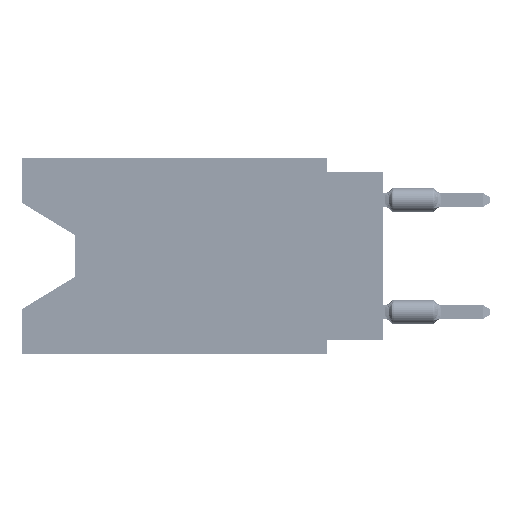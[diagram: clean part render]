
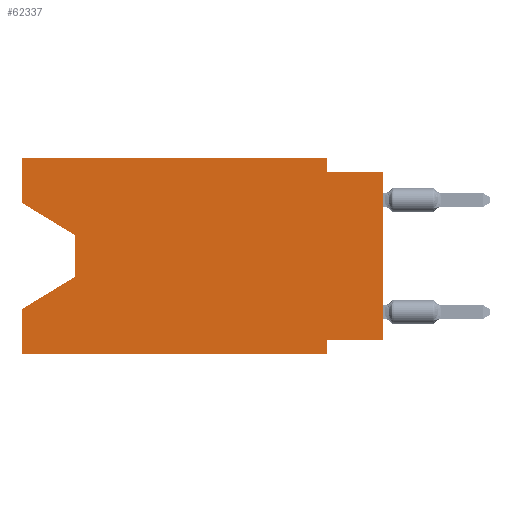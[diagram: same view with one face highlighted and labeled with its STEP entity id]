
A CAD part, left-side view. The second image highlights one B-rep face of the part: STEP entity #62337.
In plain terms, the highlighted planar face has unit normal (-1, 0, 0).
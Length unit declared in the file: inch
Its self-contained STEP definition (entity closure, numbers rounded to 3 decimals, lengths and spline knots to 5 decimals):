
#1191 = ORIENTED_EDGE ( 'NONE', *, *, #23479, .F. ) ;
#1272 = DIRECTION ( 'NONE',  ( 0., -1., 0. ) ) ;
#1857 = LINE ( 'NONE', #12989, #27364 ) ;
#2839 = LINE ( 'NONE', #30443, #30662 ) ;
#3334 = ORIENTED_EDGE ( 'NONE', *, *, #30264, .T. ) ;
#4601 = VECTOR ( 'NONE', #22509, 39.37008 ) ;
#4722 = DIRECTION ( 'NONE',  ( 0., 0., 1. ) ) ;
#5145 = ORIENTED_EDGE ( 'NONE', *, *, #39439, .F. ) ;
#5675 = CARTESIAN_POINT ( 'NONE',  ( 0., 0.55, -0.138 ) ) ;
#5821 = ORIENTED_EDGE ( 'NONE', *, *, #44535, .T. ) ;
#6218 = EDGE_CURVE ( 'NONE', #67840, #54219, #1857, .T. ) ;
#6361 = LINE ( 'NONE', #37998, #4601 ) ;
#7333 = LINE ( 'NONE', #46051, #47395 ) ;
#7729 = DIRECTION ( 'NONE',  ( 0., 0.855, -0.519 ) ) ;
#7943 = VECTOR ( 'NONE', #45613, 39.37008 ) ;
#8636 = LINE ( 'NONE', #47024, #56305 ) ;
#8919 = DIRECTION ( 'NONE',  ( 0., -1., 0. ) ) ;
#9438 = VERTEX_POINT ( 'NONE', #67692 ) ;
#9971 = ORIENTED_EDGE ( 'NONE', *, *, #41103, .F. ) ;
#10302 = CARTESIAN_POINT ( 'NONE',  ( 0., 0.1, -0.325 ) ) ;
#11143 = VECTOR ( 'NONE', #7729, 39.37008 ) ;
#12989 = CARTESIAN_POINT ( 'NONE',  ( 0., 0., -0.025 ) ) ;
#14322 = CARTESIAN_POINT ( 'NONE',  ( 0., 0.645, 0. ) ) ;
#14643 = CARTESIAN_POINT ( 'NONE',  ( 0., 0.1, -0.025 ) ) ;
#18408 = CARTESIAN_POINT ( 'NONE',  ( 0., 0.645, -0.08025 ) ) ;
#19394 = VERTEX_POINT ( 'NONE', #65000 ) ;
#20054 = DIRECTION ( 'NONE',  ( 0., 0., -1. ) ) ;
#21131 = CARTESIAN_POINT ( 'NONE',  ( 0., 0.1, 0. ) ) ;
#21195 = LINE ( 'NONE', #63802, #25116 ) ;
#21455 = LINE ( 'NONE', #53356, #33268 ) ;
#22118 = VERTEX_POINT ( 'NONE', #34055 ) ;
#22509 = DIRECTION ( 'NONE',  ( 0., 1., 0. ) ) ;
#23479 = EDGE_CURVE ( 'NONE', #62918, #26682, #6361, .T. ) ;
#23802 = CARTESIAN_POINT ( 'NONE',  ( 0., 0.645, 0. ) ) ;
#25116 = VECTOR ( 'NONE', #4722, 39.37008 ) ;
#26682 = VERTEX_POINT ( 'NONE', #10302 ) ;
#27364 = VECTOR ( 'NONE', #29454, 39.37008 ) ;
#29143 = EDGE_CURVE ( 'NONE', #19394, #67840, #36161, .T. ) ;
#29362 = VECTOR ( 'NONE', #67140, 39.37008 ) ;
#29454 = DIRECTION ( 'NONE',  ( 0., -1., 0. ) ) ;
#29942 = VERTEX_POINT ( 'NONE', #64308 ) ;
#30114 = DIRECTION ( 'NONE',  ( 0., 0., -1. ) ) ;
#30264 = EDGE_CURVE ( 'NONE', #40024, #62748, #2839, .T. ) ;
#30443 = CARTESIAN_POINT ( 'NONE',  ( 0., 0.645, -0.35 ) ) ;
#30662 = VECTOR ( 'NONE', #8919, 39.37008 ) ;
#31284 = ORIENTED_EDGE ( 'NONE', *, *, #58803, .F. ) ;
#32242 = CARTESIAN_POINT ( 'NONE',  ( 0., 0.645, -0.35 ) ) ;
#32249 = DIRECTION ( 'NONE',  ( 0., 0., -1. ) ) ;
#33268 = VECTOR ( 'NONE', #20054, 39.37008 ) ;
#33878 = VERTEX_POINT ( 'NONE', #5675 ) ;
#34055 = CARTESIAN_POINT ( 'NONE',  ( 0., 0.645, 0. ) ) ;
#34913 = LINE ( 'NONE', #23802, #58623 ) ;
#36161 = LINE ( 'NONE', #21131, #68296 ) ;
#36640 = DIRECTION ( 'NONE',  ( 0., 0., -1. ) ) ;
#37501 = ORIENTED_EDGE ( 'NONE', *, *, #63225, .F. ) ;
#37891 = ORIENTED_EDGE ( 'NONE', *, *, #43402, .T. ) ;
#37998 = CARTESIAN_POINT ( 'NONE',  ( 0., 0., -0.325 ) ) ;
#39260 = LINE ( 'NONE', #61077, #29362 ) ;
#39439 = EDGE_CURVE ( 'NONE', #40024, #61626, #21195, .T. ) ;
#40024 = VERTEX_POINT ( 'NONE', #32242 ) ;
#41103 = EDGE_CURVE ( 'NONE', #26682, #62748, #21455, .T. ) ;
#42375 = EDGE_CURVE ( 'NONE', #33878, #29942, #8636, .T. ) ;
#43402 = EDGE_CURVE ( 'NONE', #62918, #54219, #39260, .T. ) ;
#44535 = EDGE_CURVE ( 'NONE', #29942, #61626, #46114, .T. ) ;
#45613 = DIRECTION ( 'NONE',  ( 0., -0.855, -0.519 ) ) ;
#46051 = CARTESIAN_POINT ( 'NONE',  ( 0., 0.645, 0. ) ) ;
#46114 = LINE ( 'NONE', #53506, #11143 ) ;
#46610 = EDGE_LOOP ( 'NONE', ( #55899, #56020, #5821, #5145, #3334, #9971, #1191, #37891, #53678, #57524, #31284, #37501 ) ) ;
#47024 = CARTESIAN_POINT ( 'NONE',  ( 0., 0.55, -0.138 ) ) ;
#47395 = VECTOR ( 'NONE', #1272, 39.37008 ) ;
#51102 = CARTESIAN_POINT ( 'NONE',  ( 0., 0.1, -0.35 ) ) ;
#51712 = LINE ( 'NONE', #18408, #7943 ) ;
#51755 = DIRECTION ( 'NONE',  ( 0., 0., 1. ) ) ;
#53356 = CARTESIAN_POINT ( 'NONE',  ( 0., 0.1, -0.35 ) ) ;
#53506 = CARTESIAN_POINT ( 'NONE',  ( 0., 0.55, -0.212 ) ) ;
#53678 = ORIENTED_EDGE ( 'NONE', *, *, #6218, .F. ) ;
#54219 = VERTEX_POINT ( 'NONE', #67695 ) ;
#55899 = ORIENTED_EDGE ( 'NONE', *, *, #66249, .T. ) ;
#56020 = ORIENTED_EDGE ( 'NONE', *, *, #42375, .T. ) ;
#56305 = VECTOR ( 'NONE', #36640, 39.37008 ) ;
#57524 = ORIENTED_EDGE ( 'NONE', *, *, #29143, .F. ) ;
#57679 = DIRECTION ( 'NONE',  ( 1., 0., 0. ) ) ;
#58623 = VECTOR ( 'NONE', #51755, 39.37008 ) ;
#58761 = PLANE ( 'NONE',  #68171 ) ;
#58803 = EDGE_CURVE ( 'NONE', #22118, #19394, #7333, .T. ) ;
#59719 = CARTESIAN_POINT ( 'NONE',  ( 0., 0., -0.325 ) ) ;
#61077 = CARTESIAN_POINT ( 'NONE',  ( 0., 0., 0. ) ) ;
#61626 = VERTEX_POINT ( 'NONE', #63561 ) ;
#62337 = ADVANCED_FACE ( 'NONE', ( #63742 ), #58761, .F. ) ;
#62748 = VERTEX_POINT ( 'NONE', #51102 ) ;
#62918 = VERTEX_POINT ( 'NONE', #59719 ) ;
#63225 = EDGE_CURVE ( 'NONE', #9438, #22118, #34913, .T. ) ;
#63561 = CARTESIAN_POINT ( 'NONE',  ( 0., 0.645, -0.26975 ) ) ;
#63742 = FACE_OUTER_BOUND ( 'NONE', #46610, .T. ) ;
#63802 = CARTESIAN_POINT ( 'NONE',  ( 0., 0.645, 0. ) ) ;
#64308 = CARTESIAN_POINT ( 'NONE',  ( 0., 0.55, -0.212 ) ) ;
#65000 = CARTESIAN_POINT ( 'NONE',  ( 0., 0.1, 0. ) ) ;
#66249 = EDGE_CURVE ( 'NONE', #9438, #33878, #51712, .T. ) ;
#67140 = DIRECTION ( 'NONE',  ( 0., 0., 1. ) ) ;
#67692 = CARTESIAN_POINT ( 'NONE',  ( 0., 0.645, -0.08025 ) ) ;
#67695 = CARTESIAN_POINT ( 'NONE',  ( 0., 0., -0.025 ) ) ;
#67840 = VERTEX_POINT ( 'NONE', #14643 ) ;
#68171 = AXIS2_PLACEMENT_3D ( 'NONE', #14322, #57679, #30114 ) ;
#68296 = VECTOR ( 'NONE', #32249, 39.37008 ) ;
